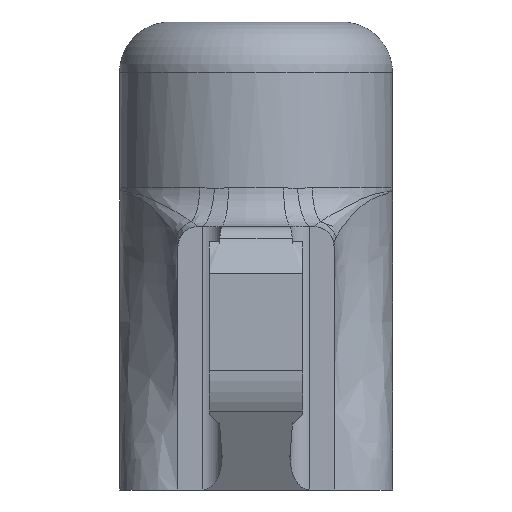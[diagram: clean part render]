
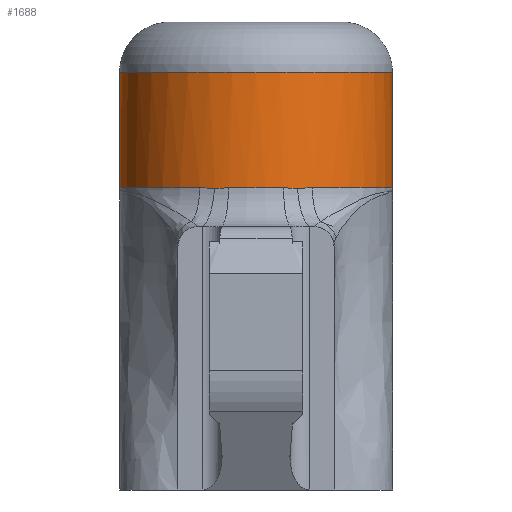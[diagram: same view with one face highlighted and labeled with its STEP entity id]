
A CAD part, front view. The second image highlights one B-rep face of the part: STEP entity #1688.
In plain terms, the highlighted cylindrical face has radius 17.5 mm (diameter 35 mm), a partial arc.
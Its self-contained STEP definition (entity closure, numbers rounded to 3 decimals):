
#7 = EDGE_CURVE ( 'NONE', #6458, #8831, #11791, .T. ) ;
#122 = EDGE_CURVE ( 'NONE', #7499, #10361, #11361, .T. ) ;
#383 = ORIENTED_EDGE ( 'NONE', *, *, #122, .T. ) ;
#434 = DIRECTION ( 'NONE',  ( 1., 0., 0. ) ) ;
#577 = ORIENTED_EDGE ( 'NONE', *, *, #7423, .T. ) ;
#837 = VERTEX_POINT ( 'NONE', #6021 ) ;
#887 = CARTESIAN_POINT ( 'NONE',  ( -17.5, 0., 53.53 ) ) ;
#1001 = DIRECTION ( 'NONE',  ( 0., 0., 1. ) ) ;
#1024 = VERTEX_POINT ( 'NONE', #2509 ) ;
#1145 = VECTOR ( 'NONE', #2190, 1000. ) ;
#1272 = VERTEX_POINT ( 'NONE', #887 ) ;
#1290 = FACE_OUTER_BOUND ( 'NONE', #11845, .T. ) ;
#1405 = AXIS2_PLACEMENT_3D ( 'NONE', #5725, #11528, #11661 ) ;
#1506 = CARTESIAN_POINT ( 'NONE',  ( 17.5, 0., 53.53 ) ) ;
#1525 = CARTESIAN_POINT ( 'NONE',  ( 4.589, -16.888, 38.677 ) ) ;
#1531 = CARTESIAN_POINT ( 'NONE',  ( 4.142, -17.006, 38.723 ) ) ;
#1688 = ADVANCED_FACE ( 'NONE', ( #1290 ), #3466, .T. ) ;
#1708 = CARTESIAN_POINT ( 'NONE',  ( -7.213, -15.944, 38.759 ) ) ;
#1718 = CARTESIAN_POINT ( 'NONE',  ( 5.332, -16.668, 38.672 ) ) ;
#1921 = CARTESIAN_POINT ( 'NONE',  ( -3.538, -17.139, 38.759 ) ) ;
#2190 = DIRECTION ( 'NONE',  ( 0., 0., -1. ) ) ;
#2356 = EDGE_CURVE ( 'NONE', #837, #9886, #5984, .T. ) ;
#2390 = CARTESIAN_POINT ( 'NONE',  ( 3.842, -17.076, 38.759 ) ) ;
#2479 = ORIENTED_EDGE ( 'NONE', *, *, #12425, .T. ) ;
#2509 = CARTESIAN_POINT ( 'NONE',  ( -17.5, 0., 38.759 ) ) ;
#2678 = CARTESIAN_POINT ( 'NONE',  ( -6.599, -16.222, 38.759 ) ) ;
#2751 = CARTESIAN_POINT ( 'NONE',  ( -3.842, -17.076, 38.759 ) ) ;
#2845 = CARTESIAN_POINT ( 'NONE',  ( -7.213, -15.944, 38.759 ) ) ;
#2939 = EDGE_CURVE ( 'NONE', #1272, #1024, #12436, .T. ) ;
#3117 = EDGE_CURVE ( 'NONE', #10361, #837, #5868, .T. ) ;
#3149 = CARTESIAN_POINT ( 'NONE',  ( -17.5, 0., 60. ) ) ;
#3466 = CYLINDRICAL_SURFACE ( 'NONE', #11779, 17.5 ) ;
#3705 = CARTESIAN_POINT ( 'NONE',  ( -4.589, -16.888, 38.677 ) ) ;
#3997 = EDGE_CURVE ( 'NONE', #8656, #7499, #8777, .T. ) ;
#4102 = CARTESIAN_POINT ( 'NONE',  ( 17.5, 0., 60. ) ) ;
#4386 = CARTESIAN_POINT ( 'NONE',  ( 0., 0., 38.759 ) ) ;
#4544 = VECTOR ( 'NONE', #10885, 1000. ) ;
#4560 = CARTESIAN_POINT ( 'NONE',  ( -5.332, -16.668, 38.672 ) ) ;
#4677 = CARTESIAN_POINT ( 'NONE',  ( -5.332, -16.668, 38.672 ) ) ;
#5313 = CIRCLE ( 'NONE', #9141, 17.5 ) ;
#5323 = LINE ( 'NONE', #4102, #4544 ) ;
#5328 = ORIENTED_EDGE ( 'NONE', *, *, #7, .T. ) ;
#5353 = DIRECTION ( 'NONE',  ( -1., 0., 0. ) ) ;
#5645 = CARTESIAN_POINT ( 'NONE',  ( -5.184, -16.715, 38.66 ) ) ;
#5685 = CARTESIAN_POINT ( 'NONE',  ( 5.035, -16.761, 38.655 ) ) ;
#5725 = CARTESIAN_POINT ( 'NONE',  ( 0., 0., 38.759 ) ) ;
#5868 = CIRCLE ( 'NONE', #7317, 17.5 ) ;
#5984 = B_SPLINE_CURVE_WITH_KNOTS ( 'NONE', 3,
 ( #7276, #2390, #1531, #1525, #7658, #5685, #11121, #1718 ),
 .UNSPECIFIED., .F., .F.,
 ( 4, 2, 2, 4 ),
 ( 0., 0.001, 0.001, 0.002 ),
 .UNSPECIFIED. ) ;
#6021 = CARTESIAN_POINT ( 'NONE',  ( 3.538, -17.139, 38.759 ) ) ;
#6062 = CARTESIAN_POINT ( 'NONE',  ( 0., 0., 60. ) ) ;
#6198 = DIRECTION ( 'NONE',  ( 0., 0., -1. ) ) ;
#6295 = CARTESIAN_POINT ( 'NONE',  ( 6.599, -16.222, 38.759 ) ) ;
#6458 = VERTEX_POINT ( 'NONE', #11168 ) ;
#6754 = CARTESIAN_POINT ( 'NONE',  ( 5.332, -16.668, 38.672 ) ) ;
#6987 = CIRCLE ( 'NONE', #7973, 17.5 ) ;
#7116 = DIRECTION ( 'NONE',  ( -1., 0., 0. ) ) ;
#7171 = ORIENTED_EDGE ( 'NONE', *, *, #2356, .T. ) ;
#7276 = CARTESIAN_POINT ( 'NONE',  ( 3.538, -17.139, 38.759 ) ) ;
#7317 = AXIS2_PLACEMENT_3D ( 'NONE', #12010, #1001, #9978 ) ;
#7423 = EDGE_CURVE ( 'NONE', #1024, #8656, #5313, .T. ) ;
#7499 = VERTEX_POINT ( 'NONE', #11274 ) ;
#7658 = CARTESIAN_POINT ( 'NONE',  ( 4.738, -16.847, 38.664 ) ) ;
#7951 = CARTESIAN_POINT ( 'NONE',  ( 17.5, 0., 38.759 ) ) ;
#7973 = AXIS2_PLACEMENT_3D ( 'NONE', #12011, #6198, #434 ) ;
#8489 = VERTEX_POINT ( 'NONE', #1506 ) ;
#8523 = ORIENTED_EDGE ( 'NONE', *, *, #3997, .T. ) ;
#8530 = CARTESIAN_POINT ( 'NONE',  ( -3.538, -17.139, 38.759 ) ) ;
#8656 = VERTEX_POINT ( 'NONE', #2845 ) ;
#8777 = B_SPLINE_CURVE_WITH_KNOTS ( 'NONE', 3,
 ( #1708, #2678, #9395, #4560 ),
 .UNSPECIFIED., .F., .F.,
 ( 4, 4 ),
 ( 0., 0.002 ),
 .UNSPECIFIED. ) ;
#8831 = VERTEX_POINT ( 'NONE', #7951 ) ;
#8982 = DIRECTION ( 'NONE',  ( 0., 0., -1. ) ) ;
#9036 = ORIENTED_EDGE ( 'NONE', *, *, #2939, .T. ) ;
#9141 = AXIS2_PLACEMENT_3D ( 'NONE', #4386, #11175, #5353 ) ;
#9183 = CARTESIAN_POINT ( 'NONE',  ( 5.332, -16.668, 38.672 ) ) ;
#9220 = CARTESIAN_POINT ( 'NONE',  ( 5.972, -16.463, 38.722 ) ) ;
#9395 = CARTESIAN_POINT ( 'NONE',  ( -5.972, -16.463, 38.722 ) ) ;
#9524 = CARTESIAN_POINT ( 'NONE',  ( -4.142, -17.006, 38.723 ) ) ;
#9556 = CARTESIAN_POINT ( 'NONE',  ( -5.035, -16.761, 38.655 ) ) ;
#9636 = ORIENTED_EDGE ( 'NONE', *, *, #10699, .F. ) ;
#9833 = EDGE_CURVE ( 'NONE', #9886, #6458, #12427, .T. ) ;
#9886 = VERTEX_POINT ( 'NONE', #9183 ) ;
#9978 = DIRECTION ( 'NONE',  ( -1., 0., 0. ) ) ;
#10361 = VERTEX_POINT ( 'NONE', #1921 ) ;
#10482 = CARTESIAN_POINT ( 'NONE',  ( -4.738, -16.847, 38.664 ) ) ;
#10699 = EDGE_CURVE ( 'NONE', #8489, #8831, #5323, .T. ) ;
#10885 = DIRECTION ( 'NONE',  ( 0., 0., -1. ) ) ;
#11121 = CARTESIAN_POINT ( 'NONE',  ( 5.184, -16.715, 38.66 ) ) ;
#11141 = CARTESIAN_POINT ( 'NONE',  ( 7.213, -15.944, 38.759 ) ) ;
#11168 = CARTESIAN_POINT ( 'NONE',  ( 7.213, -15.944, 38.759 ) ) ;
#11175 = DIRECTION ( 'NONE',  ( 0., 0., 1. ) ) ;
#11274 = CARTESIAN_POINT ( 'NONE',  ( -5.332, -16.668, 38.672 ) ) ;
#11361 = B_SPLINE_CURVE_WITH_KNOTS ( 'NONE', 3,
 ( #4677, #5645, #9556, #10482, #3705, #9524, #2751, #8530 ),
 .UNSPECIFIED., .F., .F.,
 ( 4, 2, 2, 4 ),
 ( 0., 0., 0.001, 0.002 ),
 .UNSPECIFIED. ) ;
#11450 = ORIENTED_EDGE ( 'NONE', *, *, #9833, .T. ) ;
#11528 = DIRECTION ( 'NONE',  ( 0., 0., 1. ) ) ;
#11661 = DIRECTION ( 'NONE',  ( -1., 0., 0. ) ) ;
#11779 = AXIS2_PLACEMENT_3D ( 'NONE', #6062, #8982, #7116 ) ;
#11791 = CIRCLE ( 'NONE', #1405, 17.5 ) ;
#11845 = EDGE_LOOP ( 'NONE', ( #9636, #2479, #9036, #577, #8523, #383, #11953, #7171, #11450, #5328 ) ) ;
#11953 = ORIENTED_EDGE ( 'NONE', *, *, #3117, .T. ) ;
#12010 = CARTESIAN_POINT ( 'NONE',  ( 0., 0., 38.759 ) ) ;
#12011 = CARTESIAN_POINT ( 'NONE',  ( 0., 0., 53.53 ) ) ;
#12425 = EDGE_CURVE ( 'NONE', #8489, #1272, #6987, .T. ) ;
#12427 = B_SPLINE_CURVE_WITH_KNOTS ( 'NONE', 3,
 ( #6754, #9220, #6295, #11141 ),
 .UNSPECIFIED., .F., .F.,
 ( 4, 4 ),
 ( 0., 0.002 ),
 .UNSPECIFIED. ) ;
#12436 = LINE ( 'NONE', #3149, #1145 ) ;
